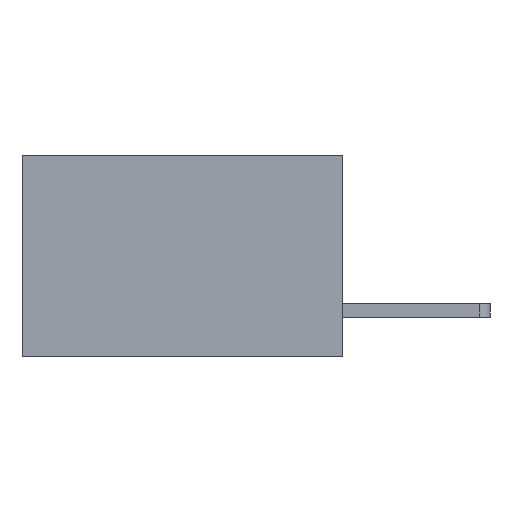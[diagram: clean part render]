
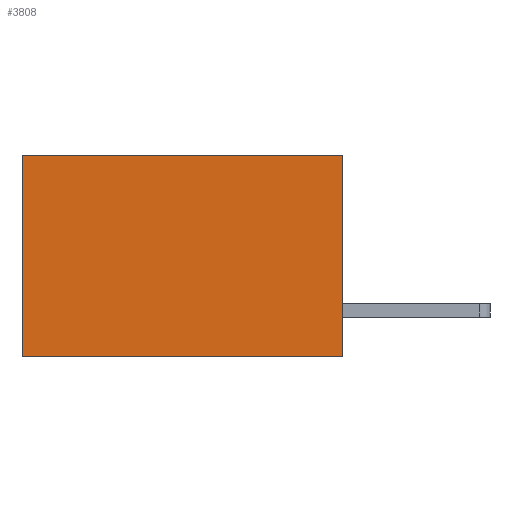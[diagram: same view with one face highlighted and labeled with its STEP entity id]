
A CAD part, left-side view. The second image highlights one B-rep face of the part: STEP entity #3808.
In plain terms, the highlighted planar face has unit normal (-1, 0, 0).
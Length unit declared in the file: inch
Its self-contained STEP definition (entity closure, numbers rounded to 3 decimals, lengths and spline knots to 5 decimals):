
#34 = CARTESIAN_POINT ( 'NONE',  ( 0.277, 0.59, -0.37 ) ) ;
#698 = CARTESIAN_POINT ( 'NONE',  ( 0.277, 0., -0.37 ) ) ;
#852 = ORIENTED_EDGE ( 'NONE', *, *, #939, .F. ) ;
#939 = EDGE_CURVE ( 'NONE', #4287, #972, #8622, .T. ) ;
#972 = VERTEX_POINT ( 'NONE', #3660 ) ;
#1132 = VERTEX_POINT ( 'NONE', #4025 ) ;
#1135 = EDGE_CURVE ( 'NONE', #1132, #4287, #6390, .T. ) ;
#1990 = DIRECTION ( 'NONE',  ( 0., 0., -1. ) ) ;
#2247 = DIRECTION ( 'NONE',  ( 0., 1., 0. ) ) ;
#2333 = EDGE_CURVE ( 'NONE', #5011, #972, #10063, .T. ) ;
#2400 = CARTESIAN_POINT ( 'NONE',  ( 0.277, 0., 0. ) ) ;
#3628 = CARTESIAN_POINT ( 'NONE',  ( 0.277, 0., -0.37 ) ) ;
#3660 = CARTESIAN_POINT ( 'NONE',  ( 0.277, 0.59, -0.37 ) ) ;
#3808 = ADVANCED_FACE ( 'NONE', ( #7346 ), #8916, .F. ) ;
#3979 = VECTOR ( 'NONE', #9350, 39.37008 ) ;
#4025 = CARTESIAN_POINT ( 'NONE',  ( 0.277, 0., 0. ) ) ;
#4133 = VECTOR ( 'NONE', #7023, 39.37008 ) ;
#4287 = VERTEX_POINT ( 'NONE', #9901 ) ;
#4796 = CARTESIAN_POINT ( 'NONE',  ( 0.277, 0., -0.37 ) ) ;
#5011 = VERTEX_POINT ( 'NONE', #5624 ) ;
#5332 = AXIS2_PLACEMENT_3D ( 'NONE', #698, #8766, #11204 ) ;
#5563 = LINE ( 'NONE', #2400, #7498 ) ;
#5624 = CARTESIAN_POINT ( 'NONE',  ( 0.277, 0.59, 0. ) ) ;
#5649 = EDGE_CURVE ( 'NONE', #1132, #5011, #5563, .T. ) ;
#5871 = EDGE_LOOP ( 'NONE', ( #9882, #852, #5890, #8035 ) ) ;
#5890 = ORIENTED_EDGE ( 'NONE', *, *, #1135, .F. ) ;
#6390 = LINE ( 'NONE', #4796, #3979 ) ;
#7023 = DIRECTION ( 'NONE',  ( 0., 1., 0. ) ) ;
#7346 = FACE_OUTER_BOUND ( 'NONE', #5871, .T. ) ;
#7498 = VECTOR ( 'NONE', #2247, 39.37008 ) ;
#7962 = VECTOR ( 'NONE', #1990, 39.37008 ) ;
#8035 = ORIENTED_EDGE ( 'NONE', *, *, #5649, .T. ) ;
#8622 = LINE ( 'NONE', #3628, #4133 ) ;
#8766 = DIRECTION ( 'NONE',  ( 1., 0., 0. ) ) ;
#8916 = PLANE ( 'NONE',  #5332 ) ;
#9350 = DIRECTION ( 'NONE',  ( 0., 0., -1. ) ) ;
#9882 = ORIENTED_EDGE ( 'NONE', *, *, #2333, .T. ) ;
#9901 = CARTESIAN_POINT ( 'NONE',  ( 0.277, 0., -0.37 ) ) ;
#10063 = LINE ( 'NONE', #34, #7962 ) ;
#11204 = DIRECTION ( 'NONE',  ( 0., 0., -1. ) ) ;
